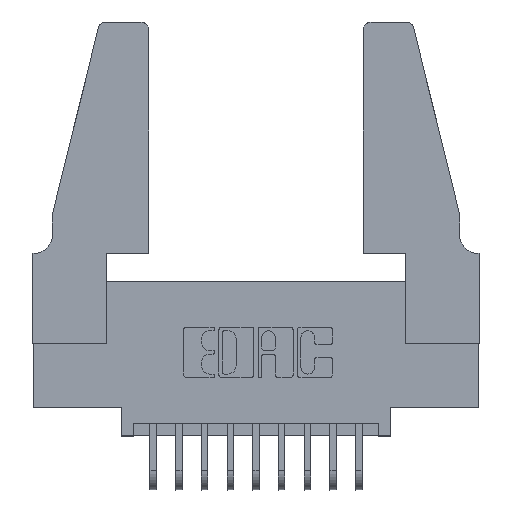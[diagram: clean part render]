
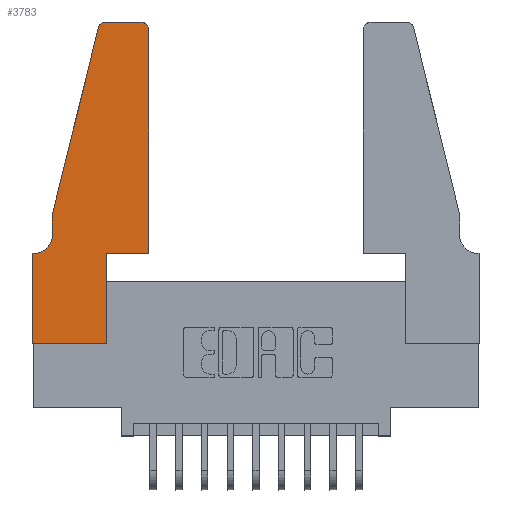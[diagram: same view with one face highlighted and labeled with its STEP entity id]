
A CAD part, top view. The second image highlights one B-rep face of the part: STEP entity #3783.
In plain terms, the highlighted planar face has unit normal (0, 0, 1).
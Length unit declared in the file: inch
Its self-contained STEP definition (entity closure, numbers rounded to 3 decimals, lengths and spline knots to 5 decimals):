
#26 = ORIENTED_EDGE ( 'NONE', *, *, #8538, .T. ) ;
#600 = VECTOR ( 'NONE', #9420, 39.37008 ) ;
#641 = AXIS2_PLACEMENT_3D ( 'NONE', #7215, #7464, #11034 ) ;
#830 = VERTEX_POINT ( 'NONE', #1016 ) ;
#967 = LINE ( 'NONE', #3029, #9399 ) ;
#1016 = CARTESIAN_POINT ( 'NONE',  ( 0.2865, 0., 0.37 ) ) ;
#1031 = VERTEX_POINT ( 'NONE', #5900 ) ;
#1122 = LINE ( 'NONE', #4000, #10825 ) ;
#1202 = CARTESIAN_POINT ( 'NONE',  ( 0.2865, 0.35, 0.37 ) ) ;
#1507 = DIRECTION ( 'NONE',  ( 0., 0., 1. ) ) ;
#1868 = CARTESIAN_POINT ( 'NONE',  ( 0.284, 1.25, 0.37 ) ) ;
#1938 = VERTEX_POINT ( 'NONE', #2655 ) ;
#1943 = VECTOR ( 'NONE', #3148, 39.37008 ) ;
#2142 = VECTOR ( 'NONE', #10303, 39.37008 ) ;
#2352 = VERTEX_POINT ( 'NONE', #8721 ) ;
#2384 = CIRCLE ( 'NONE', #641, 0.03 ) ;
#2570 = CIRCLE ( 'NONE', #13826, 0.03 ) ;
#2655 = CARTESIAN_POINT ( 'NONE',  ( 0.0755, 0.5, 0.37 ) ) ;
#2899 = CARTESIAN_POINT ( 'NONE',  ( 0.0055, 0.42, 0.37 ) ) ;
#3029 = CARTESIAN_POINT ( 'NONE',  ( 0.4505, 0.35, 0.37 ) ) ;
#3148 = DIRECTION ( 'NONE',  ( 0., -1., 0. ) ) ;
#3161 = AXIS2_PLACEMENT_3D ( 'NONE', #2899, #9029, #14790 ) ;
#3205 = CARTESIAN_POINT ( 'NONE',  ( 0.284, 1.22, 0.37 ) ) ;
#3237 = LINE ( 'NONE', #1202, #6030 ) ;
#3293 = EDGE_CURVE ( 'NONE', #1031, #7711, #15462, .T. ) ;
#3300 = ORIENTED_EDGE ( 'NONE', *, *, #5875, .T. ) ;
#3466 = CARTESIAN_POINT ( 'NONE',  ( 0., 0., 0.37 ) ) ;
#3663 = LINE ( 'NONE', #13350, #8184 ) ;
#3783 = ADVANCED_FACE ( 'NONE', ( #14496 ), #14617, .T. ) ;
#4000 = CARTESIAN_POINT ( 'NONE',  ( 0.4505, 0.35, 0.37 ) ) ;
#4028 = VERTEX_POINT ( 'NONE', #3466 ) ;
#4155 = DIRECTION ( 'NONE',  ( -1., 0., 0. ) ) ;
#4284 = ORIENTED_EDGE ( 'NONE', *, *, #14614, .T. ) ;
#4375 = LINE ( 'NONE', #7781, #2142 ) ;
#4505 = CARTESIAN_POINT ( 'NONE',  ( 0.0755, 0.42, 0.37 ) ) ;
#4853 = EDGE_CURVE ( 'NONE', #12501, #10297, #4375, .T. ) ;
#5464 = LINE ( 'NONE', #15257, #600 ) ;
#5466 = CARTESIAN_POINT ( 'NONE',  ( 0.4505, 0.35, 0.37 ) ) ;
#5560 = VERTEX_POINT ( 'NONE', #9280 ) ;
#5635 = ORIENTED_EDGE ( 'NONE', *, *, #6183, .T. ) ;
#5782 = DIRECTION ( 'NONE',  ( 1., 0., 0. ) ) ;
#5875 = EDGE_CURVE ( 'NONE', #4028, #830, #14609, .T. ) ;
#5900 = CARTESIAN_POINT ( 'NONE',  ( 0.4205, 1.25, 0.37 ) ) ;
#6030 = VECTOR ( 'NONE', #8379, 39.37008 ) ;
#6183 = EDGE_CURVE ( 'NONE', #10622, #2352, #967, .T. ) ;
#6654 = CIRCLE ( 'NONE', #3161, 0.07 ) ;
#6722 = CARTESIAN_POINT ( 'NONE',  ( 0., 0.35, 0.37 ) ) ;
#7175 = EDGE_CURVE ( 'NONE', #5560, #10622, #1122, .T. ) ;
#7215 = CARTESIAN_POINT ( 'NONE',  ( 0.4205, 1.22, 0.37 ) ) ;
#7442 = CARTESIAN_POINT ( 'NONE',  ( 0.0055, 0.35, 0.37 ) ) ;
#7464 = DIRECTION ( 'NONE',  ( 0., 0., 1. ) ) ;
#7476 = DIRECTION ( 'NONE',  ( 0., -1., 0. ) ) ;
#7580 = EDGE_CURVE ( 'NONE', #7711, #9774, #2570, .T. ) ;
#7600 = DIRECTION ( 'NONE',  ( 1., 0., 0. ) ) ;
#7659 = ORIENTED_EDGE ( 'NONE', *, *, #12835, .T. ) ;
#7711 = VERTEX_POINT ( 'NONE', #1868 ) ;
#7781 = CARTESIAN_POINT ( 'NONE',  ( 0.0755, 0.35, 0.37 ) ) ;
#7977 = CARTESIAN_POINT ( 'NONE',  ( 0.0755, 0.5, 0.37 ) ) ;
#8038 = ORIENTED_EDGE ( 'NONE', *, *, #7175, .T. ) ;
#8184 = VECTOR ( 'NONE', #7476, 39.37008 ) ;
#8379 = DIRECTION ( 'NONE',  ( 0., 1., 0. ) ) ;
#8390 = VECTOR ( 'NONE', #4155, 39.37008 ) ;
#8538 = EDGE_CURVE ( 'NONE', #2352, #1031, #2384, .T. ) ;
#8721 = CARTESIAN_POINT ( 'NONE',  ( 0.4505, 1.22, 0.37 ) ) ;
#8783 = ORIENTED_EDGE ( 'NONE', *, *, #4853, .T. ) ;
#9029 = DIRECTION ( 'NONE',  ( 0., 0., -1. ) ) ;
#9280 = CARTESIAN_POINT ( 'NONE',  ( 0.2865, 0.35, 0.37 ) ) ;
#9399 = VECTOR ( 'NONE', #13716, 39.37008 ) ;
#9420 = DIRECTION ( 'NONE',  ( -0.239, -0.971, 0. ) ) ;
#9739 = EDGE_CURVE ( 'NONE', #10297, #4028, #3663, .T. ) ;
#9774 = VERTEX_POINT ( 'NONE', #10890 ) ;
#10297 = VERTEX_POINT ( 'NONE', #11916 ) ;
#10303 = DIRECTION ( 'NONE',  ( -1., 0., 0. ) ) ;
#10437 = ORIENTED_EDGE ( 'NONE', *, *, #9739, .T. ) ;
#10547 = EDGE_CURVE ( 'NONE', #12317, #12501, #6654, .T. ) ;
#10622 = VERTEX_POINT ( 'NONE', #5466 ) ;
#10825 = VECTOR ( 'NONE', #5782, 39.37008 ) ;
#10890 = CARTESIAN_POINT ( 'NONE',  ( 0.25487, 1.22718, 0.37 ) ) ;
#11034 = DIRECTION ( 'NONE',  ( 1., 0., 0. ) ) ;
#11121 = ORIENTED_EDGE ( 'NONE', *, *, #11314, .T. ) ;
#11314 = EDGE_CURVE ( 'NONE', #1938, #12317, #12195, .T. ) ;
#11476 = ORIENTED_EDGE ( 'NONE', *, *, #7580, .T. ) ;
#11533 = DIRECTION ( 'NONE',  ( 0., 0., 1. ) ) ;
#11916 = CARTESIAN_POINT ( 'NONE',  ( 0., 0.35, 0.37 ) ) ;
#11974 = EDGE_LOOP ( 'NONE', ( #12596, #11476, #7659, #11121, #13230, #8783, #10437, #3300, #4284, #8038, #5635, #26 ) ) ;
#12034 = AXIS2_PLACEMENT_3D ( 'NONE', #6722, #1507, #7600 ) ;
#12159 = CARTESIAN_POINT ( 'NONE',  ( 0., 0., 0.37 ) ) ;
#12195 = LINE ( 'NONE', #7977, #1943 ) ;
#12317 = VERTEX_POINT ( 'NONE', #4505 ) ;
#12501 = VERTEX_POINT ( 'NONE', #7442 ) ;
#12596 = ORIENTED_EDGE ( 'NONE', *, *, #3293, .T. ) ;
#12603 = CARTESIAN_POINT ( 'NONE',  ( 0.2605, 1.25, 0.37 ) ) ;
#12740 = VECTOR ( 'NONE', #13475, 39.37008 ) ;
#12835 = EDGE_CURVE ( 'NONE', #9774, #1938, #5464, .T. ) ;
#13230 = ORIENTED_EDGE ( 'NONE', *, *, #10547, .T. ) ;
#13350 = CARTESIAN_POINT ( 'NONE',  ( 0., 0., 0.37 ) ) ;
#13475 = DIRECTION ( 'NONE',  ( 1., 0., 0. ) ) ;
#13716 = DIRECTION ( 'NONE',  ( 0., 1., 0. ) ) ;
#13826 = AXIS2_PLACEMENT_3D ( 'NONE', #3205, #11533, #13898 ) ;
#13898 = DIRECTION ( 'NONE',  ( 1., 0., 0. ) ) ;
#14496 = FACE_OUTER_BOUND ( 'NONE', #11974, .T. ) ;
#14609 = LINE ( 'NONE', #12159, #12740 ) ;
#14614 = EDGE_CURVE ( 'NONE', #830, #5560, #3237, .T. ) ;
#14617 = PLANE ( 'NONE',  #12034 ) ;
#14790 = DIRECTION ( 'NONE',  ( -1., 0., 0. ) ) ;
#15257 = CARTESIAN_POINT ( 'NONE',  ( 0.0755, 0.5, 0.37 ) ) ;
#15462 = LINE ( 'NONE', #12603, #8390 ) ;
